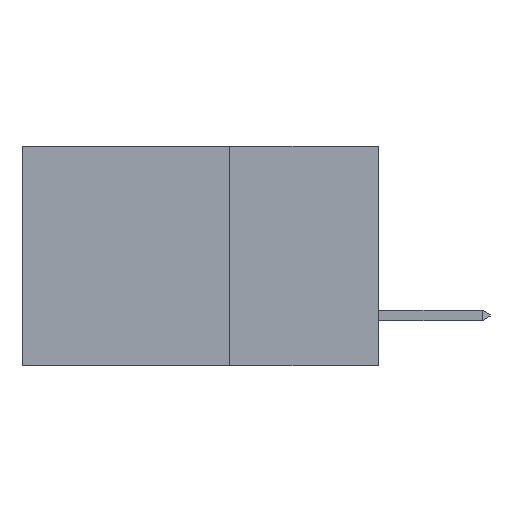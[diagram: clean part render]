
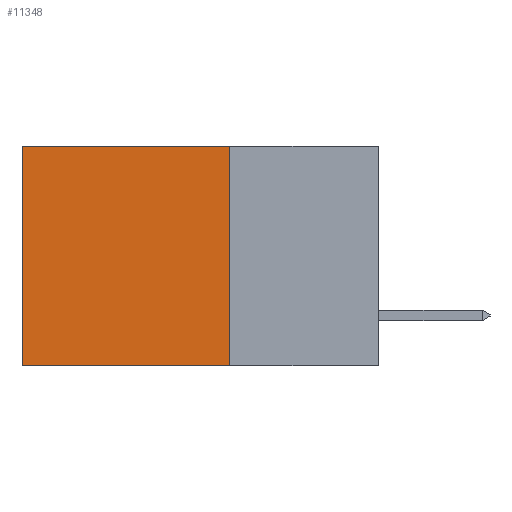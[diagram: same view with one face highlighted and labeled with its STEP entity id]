
A CAD part, left-side view. The second image highlights one B-rep face of the part: STEP entity #11348.
In plain terms, the highlighted planar face has unit normal (-1, 0, 0).
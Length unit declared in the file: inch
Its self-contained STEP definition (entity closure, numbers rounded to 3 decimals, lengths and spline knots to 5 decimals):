
#94 = LINE ( 'NONE', #13822, #3487 ) ;
#120 = ORIENTED_EDGE ( 'NONE', *, *, #13645, .F. ) ;
#508 = LINE ( 'NONE', #15375, #13074 ) ;
#983 = ORIENTED_EDGE ( 'NONE', *, *, #6497, .F. ) ;
#2628 = DIRECTION ( 'NONE',  ( 1., 0., 0. ) ) ;
#2729 = VECTOR ( 'NONE', #6355, 39.37008 ) ;
#3487 = VECTOR ( 'NONE', #14984, 39.37008 ) ;
#4581 = FACE_OUTER_BOUND ( 'NONE', #11436, .T. ) ;
#4760 = CARTESIAN_POINT ( 'NONE',  ( 0.2615, 0.6, -0.37 ) ) ;
#5130 = CARTESIAN_POINT ( 'NONE',  ( 0.2615, 0.25, -0.37 ) ) ;
#5660 = AXIS2_PLACEMENT_3D ( 'NONE', #6296, #2628, #11076 ) ;
#5835 = LINE ( 'NONE', #7832, #6566 ) ;
#6296 = CARTESIAN_POINT ( 'NONE',  ( 0.2615, 0.25, -0.37 ) ) ;
#6355 = DIRECTION ( 'NONE',  ( 0., 1., 0. ) ) ;
#6497 = EDGE_CURVE ( 'NONE', #10809, #9811, #5835, .T. ) ;
#6566 = VECTOR ( 'NONE', #7941, 39.37008 ) ;
#7054 = DIRECTION ( 'NONE',  ( 0., 1., 0. ) ) ;
#7275 = CARTESIAN_POINT ( 'NONE',  ( 0.2615, 0.6, 0. ) ) ;
#7468 = EDGE_CURVE ( 'NONE', #12545, #7763, #94, .T. ) ;
#7763 = VERTEX_POINT ( 'NONE', #4760 ) ;
#7832 = CARTESIAN_POINT ( 'NONE',  ( 0.2615, 0.25, -0.37 ) ) ;
#7941 = DIRECTION ( 'NONE',  ( 0., 0., -1. ) ) ;
#8656 = CARTESIAN_POINT ( 'NONE',  ( 0.2615, 0.25, -0.37 ) ) ;
#9697 = EDGE_CURVE ( 'NONE', #10809, #12545, #508, .T. ) ;
#9811 = VERTEX_POINT ( 'NONE', #8656 ) ;
#10809 = VERTEX_POINT ( 'NONE', #13733 ) ;
#11076 = DIRECTION ( 'NONE',  ( 0., 0., -1. ) ) ;
#11097 = ORIENTED_EDGE ( 'NONE', *, *, #9697, .T. ) ;
#11348 = ADVANCED_FACE ( 'NONE', ( #4581 ), #13460, .F. ) ;
#11436 = EDGE_LOOP ( 'NONE', ( #13334, #120, #983, #11097 ) ) ;
#12545 = VERTEX_POINT ( 'NONE', #7275 ) ;
#13074 = VECTOR ( 'NONE', #7054, 39.37008 ) ;
#13334 = ORIENTED_EDGE ( 'NONE', *, *, #7468, .T. ) ;
#13460 = PLANE ( 'NONE',  #5660 ) ;
#13645 = EDGE_CURVE ( 'NONE', #9811, #7763, #15131, .T. ) ;
#13733 = CARTESIAN_POINT ( 'NONE',  ( 0.2615, 0.25, 0. ) ) ;
#13822 = CARTESIAN_POINT ( 'NONE',  ( 0.2615, 0.6, -0.37 ) ) ;
#14984 = DIRECTION ( 'NONE',  ( 0., 0., -1. ) ) ;
#15131 = LINE ( 'NONE', #5130, #2729 ) ;
#15375 = CARTESIAN_POINT ( 'NONE',  ( 0.2615, 0.25, 0. ) ) ;
